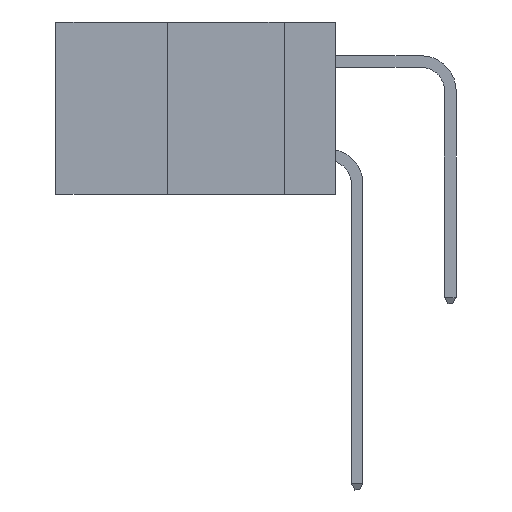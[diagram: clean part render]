
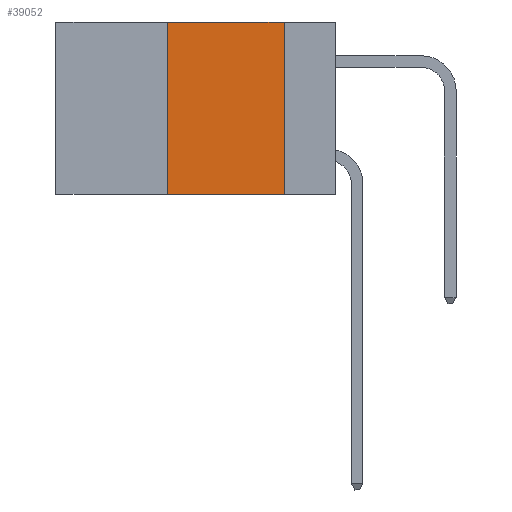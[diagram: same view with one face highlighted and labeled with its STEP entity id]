
A CAD part, left-side view. The second image highlights one B-rep face of the part: STEP entity #39052.
In plain terms, the highlighted planar face has unit normal (-1, 0, 0).
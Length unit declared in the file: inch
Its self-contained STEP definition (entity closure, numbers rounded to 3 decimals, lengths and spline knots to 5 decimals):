
#181 = DIRECTION ( 'NONE',  ( 1., 0., 0. ) ) ;
#2059 = CARTESIAN_POINT ( 'NONE',  ( 0., 0.11, 0. ) ) ;
#3336 = VECTOR ( 'NONE', #31449, 39.37008 ) ;
#3622 = DIRECTION ( 'NONE',  ( 0., -1., 0. ) ) ;
#5029 = ORIENTED_EDGE ( 'NONE', *, *, #40927, .F. ) ;
#5748 = VERTEX_POINT ( 'NONE', #31975 ) ;
#6379 = VECTOR ( 'NONE', #28954, 39.37008 ) ;
#6439 = PLANE ( 'NONE',  #19028 ) ;
#6582 = CARTESIAN_POINT ( 'NONE',  ( 0., 0.6, 0. ) ) ;
#11764 = VERTEX_POINT ( 'NONE', #35564 ) ;
#11821 = LINE ( 'NONE', #32352, #18336 ) ;
#11926 = LINE ( 'NONE', #28290, #3336 ) ;
#13480 = EDGE_CURVE ( 'NONE', #37062, #11764, #11926, .T. ) ;
#13979 = VECTOR ( 'NONE', #26464, 39.37008 ) ;
#15979 = LINE ( 'NONE', #35223, #6379 ) ;
#18336 = VECTOR ( 'NONE', #3622, 39.37008 ) ;
#19028 = AXIS2_PLACEMENT_3D ( 'NONE', #6582, #181, #22752 ) ;
#21144 = EDGE_CURVE ( 'NONE', #5748, #32351, #11821, .T. ) ;
#22333 = CARTESIAN_POINT ( 'NONE',  ( 0., 0.36, -0.37 ) ) ;
#22535 = LINE ( 'NONE', #38851, #13979 ) ;
#22752 = DIRECTION ( 'NONE',  ( 0., 0., -1. ) ) ;
#23137 = ORIENTED_EDGE ( 'NONE', *, *, #21144, .F. ) ;
#24181 = EDGE_CURVE ( 'NONE', #37062, #5748, #22535, .T. ) ;
#26464 = DIRECTION ( 'NONE',  ( 0., 0., 1. ) ) ;
#26736 = FACE_OUTER_BOUND ( 'NONE', #40642, .T. ) ;
#28290 = CARTESIAN_POINT ( 'NONE',  ( 0., 0.6, -0.37 ) ) ;
#28954 = DIRECTION ( 'NONE',  ( 0., 0., -1. ) ) ;
#30043 = ORIENTED_EDGE ( 'NONE', *, *, #13480, .T. ) ;
#31449 = DIRECTION ( 'NONE',  ( 0., -1., 0. ) ) ;
#31975 = CARTESIAN_POINT ( 'NONE',  ( 0., 0.36, 0. ) ) ;
#32351 = VERTEX_POINT ( 'NONE', #2059 ) ;
#32352 = CARTESIAN_POINT ( 'NONE',  ( 0., 0.6, 0. ) ) ;
#32464 = ORIENTED_EDGE ( 'NONE', *, *, #24181, .F. ) ;
#35223 = CARTESIAN_POINT ( 'NONE',  ( 0., 0.11, 0. ) ) ;
#35564 = CARTESIAN_POINT ( 'NONE',  ( 0., 0.11, -0.37 ) ) ;
#37062 = VERTEX_POINT ( 'NONE', #22333 ) ;
#38851 = CARTESIAN_POINT ( 'NONE',  ( 0., 0.36, 0. ) ) ;
#39052 = ADVANCED_FACE ( 'NONE', ( #26736 ), #6439, .F. ) ;
#40642 = EDGE_LOOP ( 'NONE', ( #5029, #23137, #32464, #30043 ) ) ;
#40927 = EDGE_CURVE ( 'NONE', #32351, #11764, #15979, .T. ) ;
